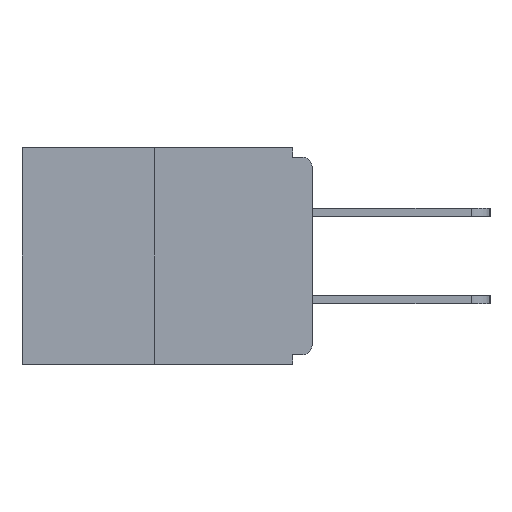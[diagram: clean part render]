
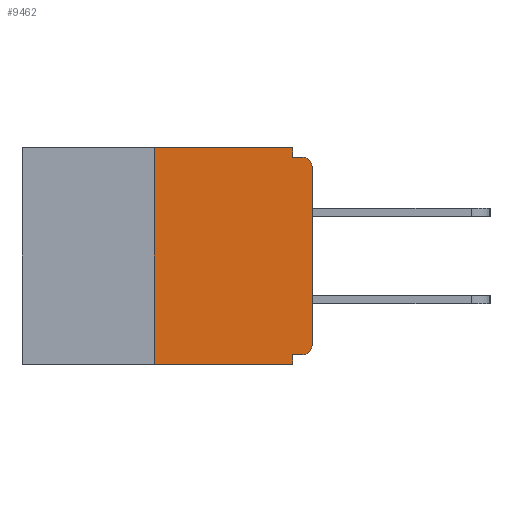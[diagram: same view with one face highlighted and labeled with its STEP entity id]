
A CAD part, left-side view. The second image highlights one B-rep face of the part: STEP entity #9462.
In plain terms, the highlighted planar face has unit normal (-1, 0, 0).
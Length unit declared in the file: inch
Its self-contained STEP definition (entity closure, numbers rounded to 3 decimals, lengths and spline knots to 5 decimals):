
#196 = VECTOR ( 'NONE', #4069, 39.37008 ) ;
#266 = ORIENTED_EDGE ( 'NONE', *, *, #4195, .F. ) ;
#1038 = VECTOR ( 'NONE', #4238, 39.37008 ) ;
#1275 = LINE ( 'NONE', #8396, #7986 ) ;
#1369 = EDGE_CURVE ( 'NONE', #2200, #2480, #5970, .T. ) ;
#1372 = LINE ( 'NONE', #15597, #1693 ) ;
#1392 = CARTESIAN_POINT ( 'NONE',  ( 0., 0.031, -0.015 ) ) ;
#1405 = ORIENTED_EDGE ( 'NONE', *, *, #1738, .T. ) ;
#1575 = VERTEX_POINT ( 'NONE', #14235 ) ;
#1579 = CARTESIAN_POINT ( 'NONE',  ( 0., 0.015, -0.015 ) ) ;
#1625 = CIRCLE ( 'NONE', #4244, 0.015 ) ;
#1693 = VECTOR ( 'NONE', #8672, 39.37008 ) ;
#1738 = EDGE_CURVE ( 'NONE', #1575, #9634, #1625, .T. ) ;
#1776 = CARTESIAN_POINT ( 'NONE',  ( 0., 0.25, 0. ) ) ;
#1973 = EDGE_LOOP ( 'NONE', ( #5505, #7881, #14746, #13890, #11223, #1405, #6200, #3766, #2681, #266 ) ) ;
#2104 = CARTESIAN_POINT ( 'NONE',  ( 0., 0.031, 0. ) ) ;
#2200 = VERTEX_POINT ( 'NONE', #15962 ) ;
#2365 = DIRECTION ( 'NONE',  ( 0., 0., -1. ) ) ;
#2402 = FACE_OUTER_BOUND ( 'NONE', #1973, .T. ) ;
#2419 = VERTEX_POINT ( 'NONE', #1776 ) ;
#2480 = VERTEX_POINT ( 'NONE', #9826 ) ;
#2681 = ORIENTED_EDGE ( 'NONE', *, *, #13145, .F. ) ;
#2889 = VERTEX_POINT ( 'NONE', #1579 ) ;
#3180 = CARTESIAN_POINT ( 'NONE',  ( 0., 0., 0. ) ) ;
#3766 = ORIENTED_EDGE ( 'NONE', *, *, #12471, .T. ) ;
#3863 = VECTOR ( 'NONE', #10878, 39.37008 ) ;
#3956 = VERTEX_POINT ( 'NONE', #1392 ) ;
#4069 = DIRECTION ( 'NONE',  ( 0., 0., 1. ) ) ;
#4195 = EDGE_CURVE ( 'NONE', #5600, #3956, #6424, .T. ) ;
#4238 = DIRECTION ( 'NONE',  ( 0., -1., 0. ) ) ;
#4244 = AXIS2_PLACEMENT_3D ( 'NONE', #12149, #10507, #2365 ) ;
#5505 = ORIENTED_EDGE ( 'NONE', *, *, #9852, .F. ) ;
#5600 = VERTEX_POINT ( 'NONE', #10742 ) ;
#5784 = CARTESIAN_POINT ( 'NONE',  ( 0., 0., -0.03 ) ) ;
#5792 = LINE ( 'NONE', #15461, #3863 ) ;
#5970 = LINE ( 'NONE', #9815, #1038 ) ;
#6200 = ORIENTED_EDGE ( 'NONE', *, *, #6785, .T. ) ;
#6424 = LINE ( 'NONE', #2104, #14428 ) ;
#6693 = EDGE_CURVE ( 'NONE', #11742, #2480, #1372, .T. ) ;
#6785 = EDGE_CURVE ( 'NONE', #9634, #7458, #8944, .T. ) ;
#7458 = VERTEX_POINT ( 'NONE', #5784 ) ;
#7476 = DIRECTION ( 'NONE',  ( 0., 0., 1. ) ) ;
#7511 = EDGE_CURVE ( 'NONE', #2200, #2419, #16582, .T. ) ;
#7668 = AXIS2_PLACEMENT_3D ( 'NONE', #13146, #15907, #10240 ) ;
#7673 = AXIS2_PLACEMENT_3D ( 'NONE', #9546, #16374, #13361 ) ;
#7684 = DIRECTION ( 'NONE',  ( 0., -1., 0. ) ) ;
#7881 = ORIENTED_EDGE ( 'NONE', *, *, #7511, .F. ) ;
#7898 = PLANE ( 'NONE',  #7673 ) ;
#7986 = VECTOR ( 'NONE', #11229, 39.37008 ) ;
#8396 = CARTESIAN_POINT ( 'NONE',  ( 0., 0., -0.015 ) ) ;
#8672 = DIRECTION ( 'NONE',  ( 0., 0., -1. ) ) ;
#8854 = LINE ( 'NONE', #14697, #16137 ) ;
#8944 = LINE ( 'NONE', #3180, #17112 ) ;
#9192 = CARTESIAN_POINT ( 'NONE',  ( 0., 0., -0.313 ) ) ;
#9413 = CARTESIAN_POINT ( 'NONE',  ( 0., 0.031, -0.328 ) ) ;
#9462 = ADVANCED_FACE ( 'NONE', ( #2402 ), #7898, .F. ) ;
#9546 = CARTESIAN_POINT ( 'NONE',  ( 0., 0.46, 0. ) ) ;
#9634 = VERTEX_POINT ( 'NONE', #9192 ) ;
#9815 = CARTESIAN_POINT ( 'NONE',  ( 0., 0.46, -0.343 ) ) ;
#9826 = CARTESIAN_POINT ( 'NONE',  ( 0., 0.031, -0.343 ) ) ;
#9852 = EDGE_CURVE ( 'NONE', #2419, #5600, #8854, .T. ) ;
#10240 = DIRECTION ( 'NONE',  ( 0., 0., -1. ) ) ;
#10507 = DIRECTION ( 'NONE',  ( -1., 0., 0. ) ) ;
#10742 = CARTESIAN_POINT ( 'NONE',  ( 0., 0.031, 0. ) ) ;
#10878 = DIRECTION ( 'NONE',  ( 0., 1., 0. ) ) ;
#11223 = ORIENTED_EDGE ( 'NONE', *, *, #11857, .F. ) ;
#11229 = DIRECTION ( 'NONE',  ( 0., -1., 0. ) ) ;
#11742 = VERTEX_POINT ( 'NONE', #9413 ) ;
#11857 = EDGE_CURVE ( 'NONE', #1575, #11742, #5792, .T. ) ;
#12149 = CARTESIAN_POINT ( 'NONE',  ( 0., 0.015, -0.313 ) ) ;
#12471 = EDGE_CURVE ( 'NONE', #7458, #2889, #16402, .T. ) ;
#13145 = EDGE_CURVE ( 'NONE', #3956, #2889, #1275, .T. ) ;
#13146 = CARTESIAN_POINT ( 'NONE',  ( 0., 0.015, -0.03 ) ) ;
#13248 = DIRECTION ( 'NONE',  ( 0., 0., -1. ) ) ;
#13361 = DIRECTION ( 'NONE',  ( 0., 0., -1. ) ) ;
#13836 = CARTESIAN_POINT ( 'NONE',  ( 0., 0.25, 0. ) ) ;
#13890 = ORIENTED_EDGE ( 'NONE', *, *, #6693, .F. ) ;
#14235 = CARTESIAN_POINT ( 'NONE',  ( 0., 0.015, -0.328 ) ) ;
#14428 = VECTOR ( 'NONE', #13248, 39.37008 ) ;
#14697 = CARTESIAN_POINT ( 'NONE',  ( 0., 0.46, 0. ) ) ;
#14746 = ORIENTED_EDGE ( 'NONE', *, *, #1369, .T. ) ;
#15461 = CARTESIAN_POINT ( 'NONE',  ( 0., 0., -0.328 ) ) ;
#15597 = CARTESIAN_POINT ( 'NONE',  ( 0., 0.031, -0.343 ) ) ;
#15907 = DIRECTION ( 'NONE',  ( -1., 0., 0. ) ) ;
#15962 = CARTESIAN_POINT ( 'NONE',  ( 0., 0.25, -0.343 ) ) ;
#16137 = VECTOR ( 'NONE', #7684, 39.37008 ) ;
#16374 = DIRECTION ( 'NONE',  ( 1., 0., 0. ) ) ;
#16402 = CIRCLE ( 'NONE', #7668, 0.015 ) ;
#16582 = LINE ( 'NONE', #13836, #196 ) ;
#17112 = VECTOR ( 'NONE', #7476, 39.37008 ) ;
